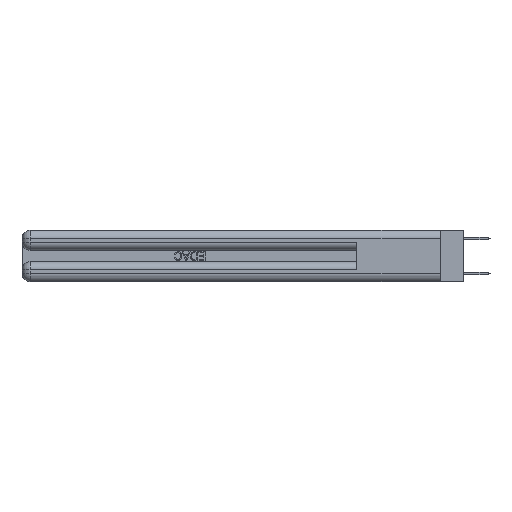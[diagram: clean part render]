
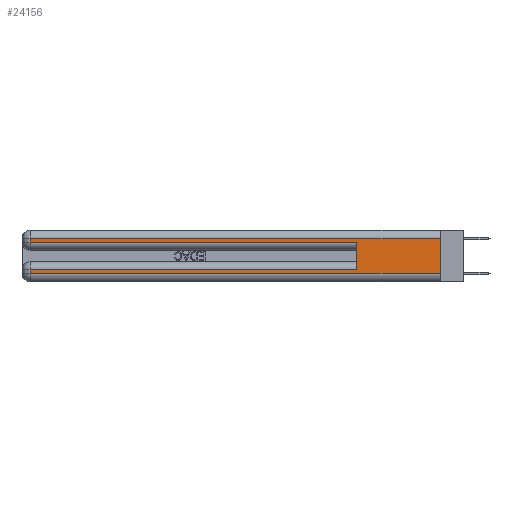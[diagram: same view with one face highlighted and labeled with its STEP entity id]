
A CAD part, left-side view. The second image highlights one B-rep face of the part: STEP entity #24156.
In plain terms, the highlighted planar face has unit normal (-1, 0, 0).
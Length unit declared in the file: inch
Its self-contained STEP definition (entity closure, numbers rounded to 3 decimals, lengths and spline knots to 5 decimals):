
#550 = ORIENTED_EDGE ( 'NONE', *, *, #645, .T. ) ;
#645 = EDGE_CURVE ( 'NONE', #12461, #3087, #8412, .T. ) ;
#977 = ORIENTED_EDGE ( 'NONE', *, *, #27770, .T. ) ;
#1062 = VECTOR ( 'NONE', #2394, 39.37008 ) ;
#1069 = LINE ( 'NONE', #7385, #33216 ) ;
#1196 = AXIS2_PLACEMENT_3D ( 'NONE', #17947, #2125, #20611 ) ;
#1365 = CARTESIAN_POINT ( 'NONE',  ( 0., 2.94, 0.37 ) ) ;
#2125 = DIRECTION ( 'NONE',  ( 1., 0., 0. ) ) ;
#2394 = DIRECTION ( 'NONE',  ( 0., -1., 0. ) ) ;
#2902 = DIRECTION ( 'NONE',  ( 0., 1., 0. ) ) ;
#3087 = VERTEX_POINT ( 'NONE', #22098 ) ;
#3102 = CARTESIAN_POINT ( 'NONE',  ( 0., 0., 0.085 ) ) ;
#3105 = CARTESIAN_POINT ( 'NONE',  ( 0., 0., 0.31 ) ) ;
#3382 = CARTESIAN_POINT ( 'NONE',  ( 0., 0., 0.37 ) ) ;
#4568 = VERTEX_POINT ( 'NONE', #33742 ) ;
#5041 = VECTOR ( 'NONE', #16564, 39.37008 ) ;
#5198 = VERTEX_POINT ( 'NONE', #28693 ) ;
#5460 = DIRECTION ( 'NONE',  ( 0., 1., 0. ) ) ;
#5597 = ORIENTED_EDGE ( 'NONE', *, *, #31208, .T. ) ;
#5984 = EDGE_CURVE ( 'NONE', #12461, #15813, #33891, .T. ) ;
#7385 = CARTESIAN_POINT ( 'NONE',  ( 0., 0., 0.06 ) ) ;
#7884 = FACE_OUTER_BOUND ( 'NONE', #17220, .T. ) ;
#8271 = CARTESIAN_POINT ( 'NONE',  ( 0., 2.94, 0.285 ) ) ;
#8412 = LINE ( 'NONE', #3102, #21591 ) ;
#8894 = VECTOR ( 'NONE', #19871, 39.37008 ) ;
#10373 = VECTOR ( 'NONE', #21336, 39.37008 ) ;
#10761 = VECTOR ( 'NONE', #5460, 39.37008 ) ;
#11326 = EDGE_CURVE ( 'NONE', #4568, #11589, #1069, .T. ) ;
#11589 = VERTEX_POINT ( 'NONE', #21535 ) ;
#11852 = CARTESIAN_POINT ( 'NONE',  ( 0., 0.6, 0.285 ) ) ;
#12461 = VERTEX_POINT ( 'NONE', #19763 ) ;
#14306 = ORIENTED_EDGE ( 'NONE', *, *, #14875, .T. ) ;
#14875 = EDGE_CURVE ( 'NONE', #3087, #4568, #22876, .T. ) ;
#15813 = VERTEX_POINT ( 'NONE', #11852 ) ;
#16132 = ORIENTED_EDGE ( 'NONE', *, *, #22534, .F. ) ;
#16490 = ORIENTED_EDGE ( 'NONE', *, *, #5984, .F. ) ;
#16564 = DIRECTION ( 'NONE',  ( 0., 0., -1. ) ) ;
#17220 = EDGE_LOOP ( 'NONE', ( #16132, #19597, #977, #5597, #16490, #550, #14306, #21387 ) ) ;
#17947 = CARTESIAN_POINT ( 'NONE',  ( 0., 0., 0.37 ) ) ;
#18683 = CARTESIAN_POINT ( 'NONE',  ( 0., 2.94, 0.37 ) ) ;
#19042 = LINE ( 'NONE', #18683, #10373 ) ;
#19093 = CARTESIAN_POINT ( 'NONE',  ( 0., 0.6, 0.145 ) ) ;
#19121 = LINE ( 'NONE', #3382, #5041 ) ;
#19597 = ORIENTED_EDGE ( 'NONE', *, *, #24292, .T. ) ;
#19763 = CARTESIAN_POINT ( 'NONE',  ( 0., 0.6, 0.085 ) ) ;
#19871 = DIRECTION ( 'NONE',  ( 0., 0., -1. ) ) ;
#20611 = DIRECTION ( 'NONE',  ( 0., 0., -1. ) ) ;
#21298 = VERTEX_POINT ( 'NONE', #8271 ) ;
#21336 = DIRECTION ( 'NONE',  ( 0., 0., -1. ) ) ;
#21387 = ORIENTED_EDGE ( 'NONE', *, *, #11326, .T. ) ;
#21535 = CARTESIAN_POINT ( 'NONE',  ( 0., 0., 0.06 ) ) ;
#21591 = VECTOR ( 'NONE', #2902, 39.37008 ) ;
#22098 = CARTESIAN_POINT ( 'NONE',  ( 0., 2.94, 0.085 ) ) ;
#22148 = LINE ( 'NONE', #33726, #1062 ) ;
#22534 = EDGE_CURVE ( 'NONE', #30067, #11589, #19121, .T. ) ;
#22876 = LINE ( 'NONE', #1365, #8894 ) ;
#23907 = CARTESIAN_POINT ( 'NONE',  ( 0., 0., 0.31 ) ) ;
#24156 = ADVANCED_FACE ( 'NONE', ( #7884 ), #25725, .F. ) ;
#24292 = EDGE_CURVE ( 'NONE', #30067, #5198, #24726, .T. ) ;
#24354 = DIRECTION ( 'NONE',  ( 0., 0., 1. ) ) ;
#24726 = LINE ( 'NONE', #23907, #10761 ) ;
#25725 = PLANE ( 'NONE',  #1196 ) ;
#27093 = VECTOR ( 'NONE', #24354, 39.37008 ) ;
#27770 = EDGE_CURVE ( 'NONE', #5198, #21298, #19042, .T. ) ;
#28368 = DIRECTION ( 'NONE',  ( 0., -1., 0. ) ) ;
#28693 = CARTESIAN_POINT ( 'NONE',  ( 0., 2.94, 0.31 ) ) ;
#30067 = VERTEX_POINT ( 'NONE', #3105 ) ;
#31208 = EDGE_CURVE ( 'NONE', #21298, #15813, #22148, .T. ) ;
#33216 = VECTOR ( 'NONE', #28368, 39.37008 ) ;
#33726 = CARTESIAN_POINT ( 'NONE',  ( 0., 0., 0.285 ) ) ;
#33742 = CARTESIAN_POINT ( 'NONE',  ( 0., 2.94, 0.06 ) ) ;
#33891 = LINE ( 'NONE', #19093, #27093 ) ;
